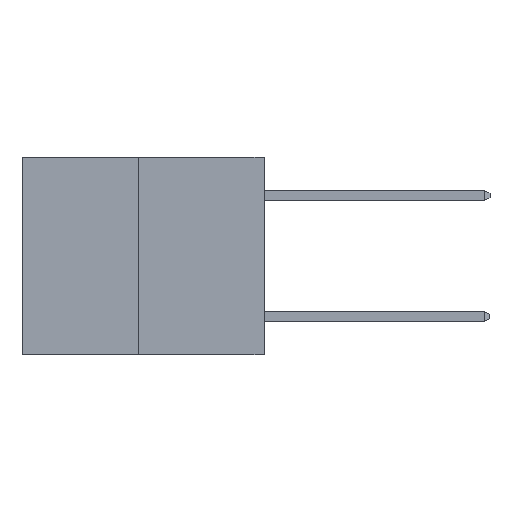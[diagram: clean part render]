
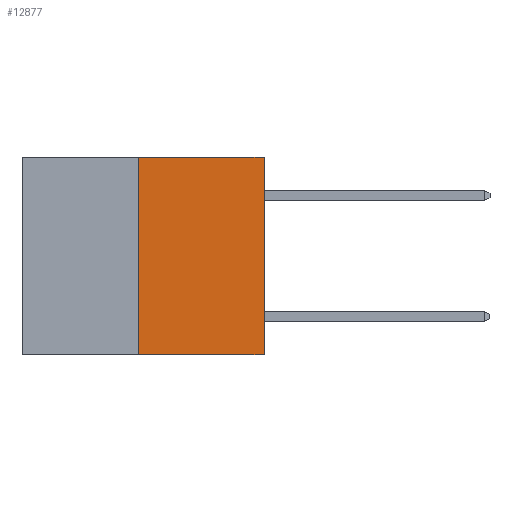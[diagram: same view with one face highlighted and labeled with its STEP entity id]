
A CAD part, left-side view. The second image highlights one B-rep face of the part: STEP entity #12877.
In plain terms, the highlighted planar face has unit normal (-1, 0, 0).
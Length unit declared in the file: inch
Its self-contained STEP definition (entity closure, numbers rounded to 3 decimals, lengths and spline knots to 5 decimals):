
#343 = DIRECTION ( 'NONE',  ( 0., -1., 0. ) ) ;
#405 = LINE ( 'NONE', #13145, #2060 ) ;
#628 = CARTESIAN_POINT ( 'NONE',  ( 0., 0.312, -0.49 ) ) ;
#948 = VECTOR ( 'NONE', #9518, 39.37008 ) ;
#1320 = VERTEX_POINT ( 'NONE', #14509 ) ;
#1406 = CARTESIAN_POINT ( 'NONE',  ( 0., 0.6, 0. ) ) ;
#1734 = EDGE_CURVE ( 'NONE', #7657, #5615, #14007, .T. ) ;
#2060 = VECTOR ( 'NONE', #343, 39.37008 ) ;
#2674 = DIRECTION ( 'NONE',  ( 0., 0., 1. ) ) ;
#3376 = LINE ( 'NONE', #15723, #9549 ) ;
#3974 = VERTEX_POINT ( 'NONE', #6976 ) ;
#5276 = CARTESIAN_POINT ( 'NONE',  ( 0., 0.312, -0.49 ) ) ;
#5535 = EDGE_CURVE ( 'NONE', #1320, #3974, #3376, .T. ) ;
#5615 = VERTEX_POINT ( 'NONE', #12233 ) ;
#6134 = ORIENTED_EDGE ( 'NONE', *, *, #1734, .F. ) ;
#6490 = DIRECTION ( 'NONE',  ( 1., 0., 0. ) ) ;
#6976 = CARTESIAN_POINT ( 'NONE',  ( 0., 0., 0. ) ) ;
#7585 = EDGE_CURVE ( 'NONE', #7657, #1320, #16300, .T. ) ;
#7657 = VERTEX_POINT ( 'NONE', #628 ) ;
#7795 = DIRECTION ( 'NONE',  ( 0., 0., -1. ) ) ;
#9518 = DIRECTION ( 'NONE',  ( 0., -1., 0. ) ) ;
#9549 = VECTOR ( 'NONE', #2674, 39.37008 ) ;
#10398 = ORIENTED_EDGE ( 'NONE', *, *, #5535, .T. ) ;
#11076 = EDGE_CURVE ( 'NONE', #5615, #3974, #405, .T. ) ;
#11723 = DIRECTION ( 'NONE',  ( 0., 0., 1. ) ) ;
#11790 = PLANE ( 'NONE',  #13435 ) ;
#11976 = CARTESIAN_POINT ( 'NONE',  ( 0., 0.6, -0.49 ) ) ;
#12233 = CARTESIAN_POINT ( 'NONE',  ( 0., 0.312, 0. ) ) ;
#12430 = ORIENTED_EDGE ( 'NONE', *, *, #11076, .F. ) ;
#12877 = ADVANCED_FACE ( 'NONE', ( #14508 ), #11790, .F. ) ;
#13145 = CARTESIAN_POINT ( 'NONE',  ( 0., 0.6, 0. ) ) ;
#13435 = AXIS2_PLACEMENT_3D ( 'NONE', #1406, #6490, #7795 ) ;
#14007 = LINE ( 'NONE', #5276, #14598 ) ;
#14508 = FACE_OUTER_BOUND ( 'NONE', #14852, .T. ) ;
#14509 = CARTESIAN_POINT ( 'NONE',  ( 0., 0., -0.49 ) ) ;
#14598 = VECTOR ( 'NONE', #11723, 39.37008 ) ;
#14852 = EDGE_LOOP ( 'NONE', ( #6134, #15131, #10398, #12430 ) ) ;
#15131 = ORIENTED_EDGE ( 'NONE', *, *, #7585, .T. ) ;
#15723 = CARTESIAN_POINT ( 'NONE',  ( 0., 0., 0. ) ) ;
#16300 = LINE ( 'NONE', #11976, #948 ) ;
